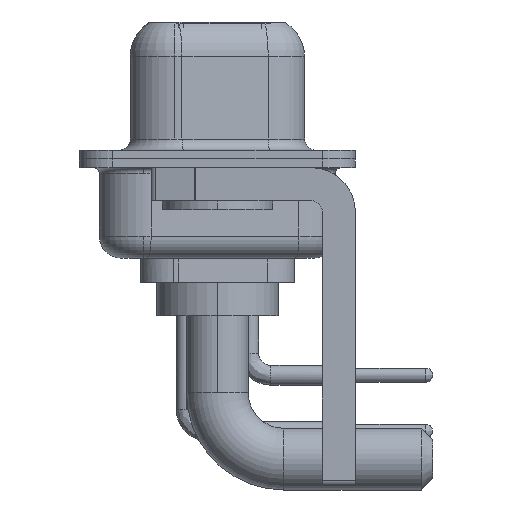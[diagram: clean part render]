
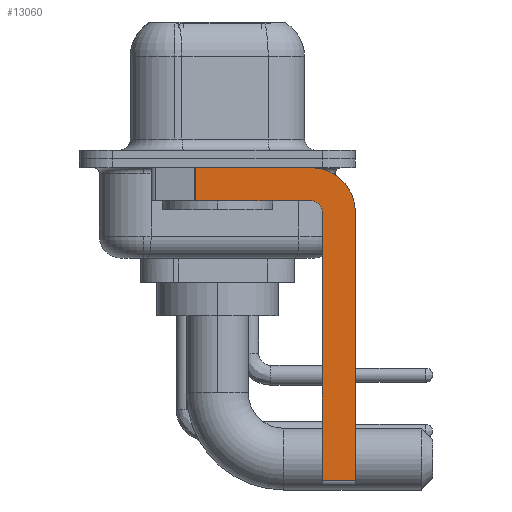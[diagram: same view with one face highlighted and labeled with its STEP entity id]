
A CAD part, left-side view. The second image highlights one B-rep face of the part: STEP entity #13060.
In plain terms, the highlighted planar face has unit normal (-1, 0, 0).
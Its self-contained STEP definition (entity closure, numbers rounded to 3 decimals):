
#13 = CARTESIAN_POINT ( 'NONE',  ( -2.9, -4.25, -2.4 ) ) ;
#99 = VECTOR ( 'NONE', #8519, 1000. ) ;
#600 = DIRECTION ( 'NONE',  ( 0., -1., 0. ) ) ;
#831 = CARTESIAN_POINT ( 'NONE',  ( -2.9, 0.978, -1.9 ) ) ;
#967 = CARTESIAN_POINT ( 'NONE',  ( -2.9, 0.978, -1.9 ) ) ;
#991 = PLANE ( 'NONE',  #8526 ) ;
#1194 = ORIENTED_EDGE ( 'NONE', *, *, #14913, .T. ) ;
#1360 = ORIENTED_EDGE ( 'NONE', *, *, #14053, .F. ) ;
#1717 = CARTESIAN_POINT ( 'NONE',  ( -2.9, -4.25, -0.4 ) ) ;
#1804 = CARTESIAN_POINT ( 'NONE',  ( -2.9, -4.25, -2.4 ) ) ;
#1896 = EDGE_LOOP ( 'NONE', ( #7728, #1194, #8226, #11650, #1360, #20339, #16587, #12483 ) ) ;
#2719 = VERTEX_POINT ( 'NONE', #18486 ) ;
#2803 = CARTESIAN_POINT ( 'NONE',  ( -2.9, -4.25, -1.9 ) ) ;
#3081 = EDGE_CURVE ( 'NONE', #7681, #15847, #11786, .T. ) ;
#3238 = CARTESIAN_POINT ( 'NONE',  ( -2.9, -6.25, -2.4 ) ) ;
#4175 = AXIS2_PLACEMENT_3D ( 'NONE', #1804, #5260, #8835 ) ;
#5260 = DIRECTION ( 'NONE',  ( -1., 0., 0. ) ) ;
#6173 = CARTESIAN_POINT ( 'NONE',  ( -2.9, -4.25, -2.4 ) ) ;
#6235 = CARTESIAN_POINT ( 'NONE',  ( -2.9, -4.25, -14.55 ) ) ;
#6288 = FACE_OUTER_BOUND ( 'NONE', #1896, .T. ) ;
#7037 = DIRECTION ( 'NONE',  ( 1., 0., 0. ) ) ;
#7190 = CARTESIAN_POINT ( 'NONE',  ( -2.9, -6.25, -2.4 ) ) ;
#7424 = VERTEX_POINT ( 'NONE', #7701 ) ;
#7681 = VERTEX_POINT ( 'NONE', #20498 ) ;
#7701 = CARTESIAN_POINT ( 'NONE',  ( -2.9, 0.978, -0.4 ) ) ;
#7728 = ORIENTED_EDGE ( 'NONE', *, *, #21737, .F. ) ;
#7799 = VERTEX_POINT ( 'NONE', #10695 ) ;
#8226 = ORIENTED_EDGE ( 'NONE', *, *, #3081, .F. ) ;
#8281 = LINE ( 'NONE', #17027, #99 ) ;
#8479 = VERTEX_POINT ( 'NONE', #3238 ) ;
#8519 = DIRECTION ( 'NONE',  ( 0., 0., 1. ) ) ;
#8526 = AXIS2_PLACEMENT_3D ( 'NONE', #6173, #11594, #12878 ) ;
#8835 = DIRECTION ( 'NONE',  ( 0., 0., 1. ) ) ;
#9165 = DIRECTION ( 'NONE',  ( 0., 0., -1. ) ) ;
#9715 = DIRECTION ( 'NONE',  ( 0., 1., 0. ) ) ;
#9735 = DIRECTION ( 'NONE',  ( 0., 0., -1. ) ) ;
#10518 = AXIS2_PLACEMENT_3D ( 'NONE', #13, #7037, #19367 ) ;
#10695 = CARTESIAN_POINT ( 'NONE',  ( -2.9, -6.25, -14.55 ) ) ;
#11001 = EDGE_CURVE ( 'NONE', #14119, #8479, #20446, .T. ) ;
#11432 = LINE ( 'NONE', #6235, #13750 ) ;
#11594 = DIRECTION ( 'NONE',  ( 1., 0., 0. ) ) ;
#11650 = ORIENTED_EDGE ( 'NONE', *, *, #14832, .F. ) ;
#11786 = LINE ( 'NONE', #2803, #17140 ) ;
#12483 = ORIENTED_EDGE ( 'NONE', *, *, #11001, .F. ) ;
#12878 = DIRECTION ( 'NONE',  ( 0., 0., -1. ) ) ;
#13004 = CIRCLE ( 'NONE', #4175, 0.5 ) ;
#13060 = ADVANCED_FACE ( 'NONE', ( #6288 ), #991, .F. ) ;
#13272 = CARTESIAN_POINT ( 'NONE',  ( -2.9, -4.75, -2.4 ) ) ;
#13750 = VECTOR ( 'NONE', #600, 1000. ) ;
#14053 = EDGE_CURVE ( 'NONE', #2719, #17336, #8281, .T. ) ;
#14119 = VERTEX_POINT ( 'NONE', #1717 ) ;
#14832 = EDGE_CURVE ( 'NONE', #17336, #7681, #13004, .T. ) ;
#14913 = EDGE_CURVE ( 'NONE', #7424, #15847, #18149, .T. ) ;
#15428 = EDGE_CURVE ( 'NONE', #2719, #7799, #11432, .T. ) ;
#15847 = VERTEX_POINT ( 'NONE', #831 ) ;
#16587 = ORIENTED_EDGE ( 'NONE', *, *, #19056, .F. ) ;
#16776 = VECTOR ( 'NONE', #9165, 1000. ) ;
#17027 = CARTESIAN_POINT ( 'NONE',  ( -2.9, -4.75, -14.8 ) ) ;
#17140 = VECTOR ( 'NONE', #9715, 1000. ) ;
#17336 = VERTEX_POINT ( 'NONE', #13272 ) ;
#18149 = LINE ( 'NONE', #967, #19621 ) ;
#18376 = VECTOR ( 'NONE', #22238, 1000. ) ;
#18486 = CARTESIAN_POINT ( 'NONE',  ( -2.9, -4.75, -14.55 ) ) ;
#18543 = LINE ( 'NONE', #22363, #18376 ) ;
#19056 = EDGE_CURVE ( 'NONE', #8479, #7799, #19528, .T. ) ;
#19367 = DIRECTION ( 'NONE',  ( 0., 0., -1. ) ) ;
#19528 = LINE ( 'NONE', #7190, #16776 ) ;
#19621 = VECTOR ( 'NONE', #9735, 1000. ) ;
#20339 = ORIENTED_EDGE ( 'NONE', *, *, #15428, .T. ) ;
#20446 = CIRCLE ( 'NONE', #10518, 2. ) ;
#20498 = CARTESIAN_POINT ( 'NONE',  ( -2.9, -4.25, -1.9 ) ) ;
#21737 = EDGE_CURVE ( 'NONE', #7424, #14119, #18543, .T. ) ;
#22238 = DIRECTION ( 'NONE',  ( 0., -1., 0. ) ) ;
#22363 = CARTESIAN_POINT ( 'NONE',  ( -2.9, 3., -0.4 ) ) ;
